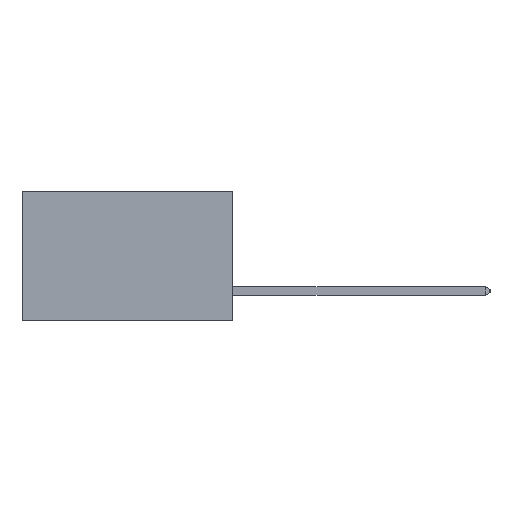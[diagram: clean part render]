
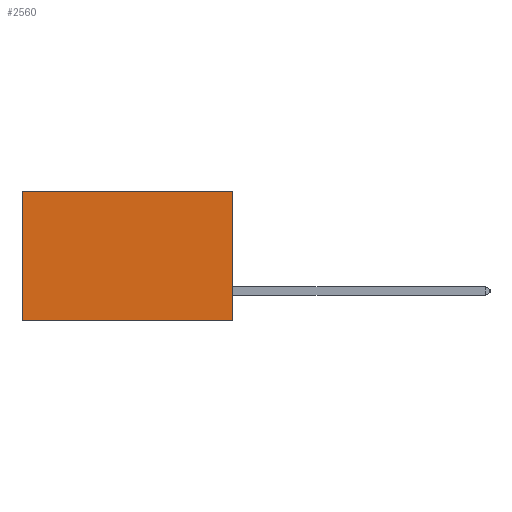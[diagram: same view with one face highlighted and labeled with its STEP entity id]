
A CAD part, left-side view. The second image highlights one B-rep face of the part: STEP entity #2560.
In plain terms, the highlighted planar face has unit normal (-1, 0, 0).
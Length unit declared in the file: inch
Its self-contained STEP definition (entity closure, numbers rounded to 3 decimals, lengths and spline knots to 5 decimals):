
#868 = VECTOR ( 'NONE', #14212, 39.37008 ) ;
#889 = DIRECTION ( 'NONE',  ( 1., 0., 0. ) ) ;
#996 = CARTESIAN_POINT ( 'NONE',  ( 0.2875, 0.6, 0. ) ) ;
#1051 = CARTESIAN_POINT ( 'NONE',  ( 0.2875, 0., -0.37 ) ) ;
#1675 = LINE ( 'NONE', #8914, #868 ) ;
#1789 = ORIENTED_EDGE ( 'NONE', *, *, #5619, .F. ) ;
#2174 = CARTESIAN_POINT ( 'NONE',  ( 0.2875, 0., 0. ) ) ;
#2275 = CARTESIAN_POINT ( 'NONE',  ( 0.2875, 0., 0. ) ) ;
#2560 = ADVANCED_FACE ( 'NONE', ( #3481 ), #5688, .F. ) ;
#2585 = VECTOR ( 'NONE', #3546, 39.37008 ) ;
#2603 = VERTEX_POINT ( 'NONE', #1051 ) ;
#3366 = LINE ( 'NONE', #2275, #2585 ) ;
#3450 = DIRECTION ( 'NONE',  ( 0., 1., 0. ) ) ;
#3481 = FACE_OUTER_BOUND ( 'NONE', #4064, .T. ) ;
#3546 = DIRECTION ( 'NONE',  ( 0., 0., -1. ) ) ;
#4064 = EDGE_LOOP ( 'NONE', ( #7570, #7004, #1789, #12375 ) ) ;
#4067 = VERTEX_POINT ( 'NONE', #9324 ) ;
#4535 = CARTESIAN_POINT ( 'NONE',  ( 0.2875, 0., 0. ) ) ;
#5175 = CARTESIAN_POINT ( 'NONE',  ( 0.2875, 0., 0. ) ) ;
#5285 = VERTEX_POINT ( 'NONE', #996 ) ;
#5554 = EDGE_CURVE ( 'NONE', #9221, #5285, #7834, .T. ) ;
#5619 = EDGE_CURVE ( 'NONE', #9221, #2603, #3366, .T. ) ;
#5688 = PLANE ( 'NONE',  #14098 ) ;
#7004 = ORIENTED_EDGE ( 'NONE', *, *, #11196, .F. ) ;
#7570 = ORIENTED_EDGE ( 'NONE', *, *, #12688, .T. ) ;
#7834 = LINE ( 'NONE', #2174, #12918 ) ;
#7961 = DIRECTION ( 'NONE',  ( 0., 0., -1. ) ) ;
#8914 = CARTESIAN_POINT ( 'NONE',  ( 0.2875, 0., -0.37 ) ) ;
#9221 = VERTEX_POINT ( 'NONE', #5175 ) ;
#9324 = CARTESIAN_POINT ( 'NONE',  ( 0.2875, 0.6, -0.37 ) ) ;
#11196 = EDGE_CURVE ( 'NONE', #2603, #4067, #1675, .T. ) ;
#12375 = ORIENTED_EDGE ( 'NONE', *, *, #5554, .T. ) ;
#12688 = EDGE_CURVE ( 'NONE', #5285, #4067, #13174, .T. ) ;
#12704 = CARTESIAN_POINT ( 'NONE',  ( 0.2875, 0.6, 0. ) ) ;
#12852 = VECTOR ( 'NONE', #13690, 39.37008 ) ;
#12918 = VECTOR ( 'NONE', #3450, 39.37008 ) ;
#13174 = LINE ( 'NONE', #12704, #12852 ) ;
#13690 = DIRECTION ( 'NONE',  ( 0., 0., -1. ) ) ;
#14098 = AXIS2_PLACEMENT_3D ( 'NONE', #4535, #889, #7961 ) ;
#14212 = DIRECTION ( 'NONE',  ( 0., 1., 0. ) ) ;
